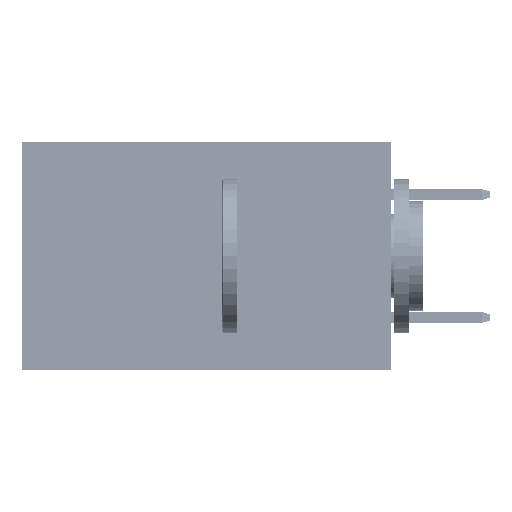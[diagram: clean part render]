
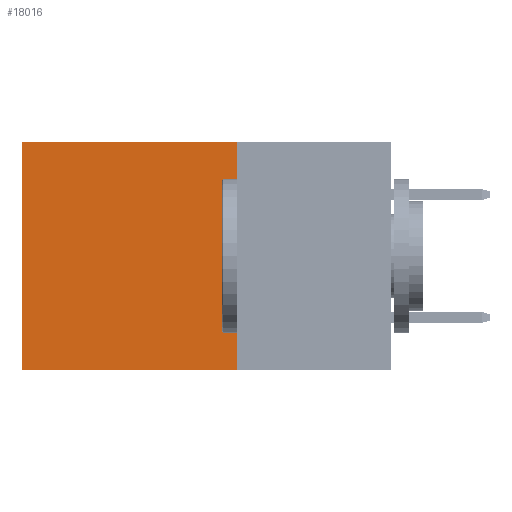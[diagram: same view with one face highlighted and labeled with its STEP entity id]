
A CAD part, left-side view. The second image highlights one B-rep face of the part: STEP entity #18016.
In plain terms, the highlighted planar face has unit normal (-1, 0, 0).
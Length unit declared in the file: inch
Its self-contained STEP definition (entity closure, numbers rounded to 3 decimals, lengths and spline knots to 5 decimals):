
#382 = FACE_OUTER_BOUND ( 'NONE', #31404, .T. ) ;
#2585 = VECTOR ( 'NONE', #12514, 39.37008 ) ;
#5394 = AXIS2_PLACEMENT_3D ( 'NONE', #28205, #44380, #8000 ) ;
#5424 = CARTESIAN_POINT ( 'NONE',  ( 0.2875, 0.6, 0. ) ) ;
#6058 = ORIENTED_EDGE ( 'NONE', *, *, #40502, .T. ) ;
#6539 = CARTESIAN_POINT ( 'NONE',  ( 0.2875, 0.25, 0. ) ) ;
#7294 = LINE ( 'NONE', #6539, #47283 ) ;
#8000 = DIRECTION ( 'NONE',  ( 0., 0., -1. ) ) ;
#8347 = EDGE_CURVE ( 'NONE', #26467, #49834, #40685, .T. ) ;
#12514 = DIRECTION ( 'NONE',  ( 0., 1., 0. ) ) ;
#16146 = ORIENTED_EDGE ( 'NONE', *, *, #8347, .F. ) ;
#18016 = ADVANCED_FACE ( 'NONE', ( #382 ), #23793, .F. ) ;
#18352 = CARTESIAN_POINT ( 'NONE',  ( 0.2875, 0.25, -0.37 ) ) ;
#18745 = CARTESIAN_POINT ( 'NONE',  ( 0.2875, 0.25, 0. ) ) ;
#22432 = LINE ( 'NONE', #18745, #36946 ) ;
#22790 = LINE ( 'NONE', #43113, #42510 ) ;
#23793 = PLANE ( 'NONE',  #5394 ) ;
#24574 = VERTEX_POINT ( 'NONE', #5424 ) ;
#24707 = CARTESIAN_POINT ( 'NONE',  ( 0.2875, 0.25, -0.37 ) ) ;
#25941 = VERTEX_POINT ( 'NONE', #41978 ) ;
#26467 = VERTEX_POINT ( 'NONE', #18352 ) ;
#26930 = DIRECTION ( 'NONE',  ( 0., 0., -1. ) ) ;
#28205 = CARTESIAN_POINT ( 'NONE',  ( 0.2875, 0.25, 0. ) ) ;
#31404 = EDGE_LOOP ( 'NONE', ( #6058, #16146, #42530, #42029 ) ) ;
#36946 = VECTOR ( 'NONE', #50677, 39.37008 ) ;
#40502 = EDGE_CURVE ( 'NONE', #24574, #49834, #22790, .T. ) ;
#40685 = LINE ( 'NONE', #24707, #2585 ) ;
#41978 = CARTESIAN_POINT ( 'NONE',  ( 0.2875, 0.25, 0. ) ) ;
#42029 = ORIENTED_EDGE ( 'NONE', *, *, #46028, .T. ) ;
#42510 = VECTOR ( 'NONE', #26930, 39.37008 ) ;
#42530 = ORIENTED_EDGE ( 'NONE', *, *, #51400, .F. ) ;
#43113 = CARTESIAN_POINT ( 'NONE',  ( 0.2875, 0.6, 0. ) ) ;
#44380 = DIRECTION ( 'NONE',  ( 1., 0., 0. ) ) ;
#46028 = EDGE_CURVE ( 'NONE', #25941, #24574, #22432, .T. ) ;
#47283 = VECTOR ( 'NONE', #51415, 39.37008 ) ;
#49834 = VERTEX_POINT ( 'NONE', #50857 ) ;
#50677 = DIRECTION ( 'NONE',  ( 0., 1., 0. ) ) ;
#50857 = CARTESIAN_POINT ( 'NONE',  ( 0.2875, 0.6, -0.37 ) ) ;
#51400 = EDGE_CURVE ( 'NONE', #25941, #26467, #7294, .T. ) ;
#51415 = DIRECTION ( 'NONE',  ( 0., 0., -1. ) ) ;
